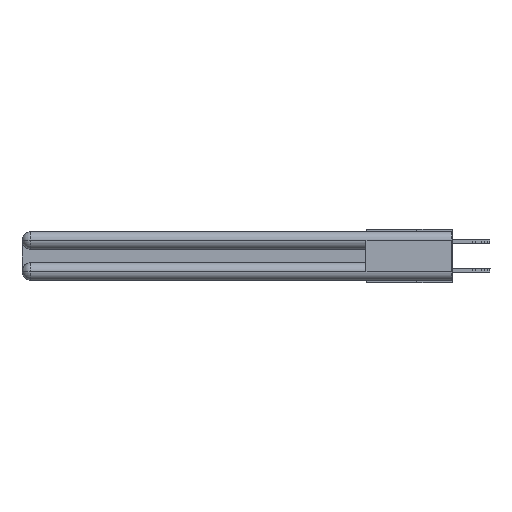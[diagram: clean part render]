
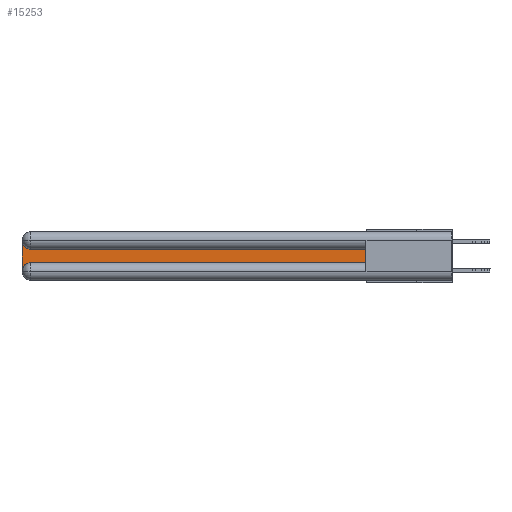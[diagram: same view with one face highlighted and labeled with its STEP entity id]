
A CAD part, left-side view. The second image highlights one B-rep face of the part: STEP entity #15253.
In plain terms, the highlighted planar face has unit normal (-1, 0, 0).
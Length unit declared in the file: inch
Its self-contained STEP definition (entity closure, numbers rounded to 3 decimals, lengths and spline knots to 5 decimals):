
#932 = CARTESIAN_POINT ( 'NONE',  ( 0.075, 2.94, -0.2775 ) ) ;
#955 = PLANE ( 'NONE',  #4731 ) ;
#1133 = EDGE_CURVE ( 'NONE', #23090, #23744, #9291, .T. ) ;
#1704 = LINE ( 'NONE', #3527, #16113 ) ;
#1966 = DIRECTION ( 'NONE',  ( 1., 0., 0. ) ) ;
#3527 = CARTESIAN_POINT ( 'NONE',  ( 0.075, 3., -0.2175 ) ) ;
#3619 = DIRECTION ( 'NONE',  ( 0., 1., 0. ) ) ;
#3834 = CARTESIAN_POINT ( 'NONE',  ( 0.075, 0.6, -0.2175 ) ) ;
#4066 = VERTEX_POINT ( 'NONE', #31238 ) ;
#4229 = VECTOR ( 'NONE', #23165, 39.37008 ) ;
#4731 = AXIS2_PLACEMENT_3D ( 'NONE', #6614, #17396, #9209 ) ;
#5042 = CARTESIAN_POINT ( 'NONE',  ( 0.075, 2.94, -0.1225 ) ) ;
#6614 = CARTESIAN_POINT ( 'NONE',  ( 0.075, 3., -0.1225 ) ) ;
#7005 = VERTEX_POINT ( 'NONE', #5042 ) ;
#7265 = CARTESIAN_POINT ( 'NONE',  ( 0.075, 2.94, -0.0625 ) ) ;
#7665 = AXIS2_PLACEMENT_3D ( 'NONE', #932, #22850, #22621 ) ;
#8088 = VECTOR ( 'NONE', #17691, 39.37008 ) ;
#8724 = EDGE_CURVE ( 'NONE', #25640, #23090, #16023, .T. ) ;
#9209 = DIRECTION ( 'NONE',  ( 0., 0., -1. ) ) ;
#9291 = LINE ( 'NONE', #9478, #4229 ) ;
#9478 = CARTESIAN_POINT ( 'NONE',  ( 0.075, 0.6, -0.2175 ) ) ;
#14307 = VERTEX_POINT ( 'NONE', #34227 ) ;
#14791 = ORIENTED_EDGE ( 'NONE', *, *, #8724, .T. ) ;
#15253 = ADVANCED_FACE ( 'NONE', ( #20458 ), #955, .F. ) ;
#16023 = CIRCLE ( 'NONE', #7665, 0.06 ) ;
#16113 = VECTOR ( 'NONE', #22501, 39.37008 ) ;
#17396 = DIRECTION ( 'NONE',  ( 1., 0., 0. ) ) ;
#17691 = DIRECTION ( 'NONE',  ( 0., 0., 1. ) ) ;
#18171 = ORIENTED_EDGE ( 'NONE', *, *, #1133, .T. ) ;
#19861 = ORIENTED_EDGE ( 'NONE', *, *, #34263, .T. ) ;
#20234 = CARTESIAN_POINT ( 'NONE',  ( 0.075, 0.6, -0.1225 ) ) ;
#20382 = EDGE_LOOP ( 'NONE', ( #28354, #23493, #34566, #14791, #18171, #19861 ) ) ;
#20458 = FACE_OUTER_BOUND ( 'NONE', #20382, .T. ) ;
#20697 = CARTESIAN_POINT ( 'NONE',  ( 0.075, 2.94, -0.2175 ) ) ;
#21465 = CARTESIAN_POINT ( 'NONE',  ( 0.075, 0.6, -0.2175 ) ) ;
#22501 = DIRECTION ( 'NONE',  ( 0., 0., -1. ) ) ;
#22621 = DIRECTION ( 'NONE',  ( 0., 0., -1. ) ) ;
#22850 = DIRECTION ( 'NONE',  ( 1., 0., 0. ) ) ;
#23090 = VERTEX_POINT ( 'NONE', #20697 ) ;
#23165 = DIRECTION ( 'NONE',  ( 0., -1., 0. ) ) ;
#23493 = ORIENTED_EDGE ( 'NONE', *, *, #26730, .T. ) ;
#23744 = VERTEX_POINT ( 'NONE', #21465 ) ;
#24038 = LINE ( 'NONE', #20234, #27482 ) ;
#25271 = CIRCLE ( 'NONE', #31290, 0.06 ) ;
#25640 = VERTEX_POINT ( 'NONE', #32980 ) ;
#26730 = EDGE_CURVE ( 'NONE', #7005, #14307, #25271, .T. ) ;
#27482 = VECTOR ( 'NONE', #3619, 39.37008 ) ;
#28354 = ORIENTED_EDGE ( 'NONE', *, *, #31181, .T. ) ;
#29781 = LINE ( 'NONE', #3834, #8088 ) ;
#31181 = EDGE_CURVE ( 'NONE', #4066, #7005, #24038, .T. ) ;
#31238 = CARTESIAN_POINT ( 'NONE',  ( 0.075, 0.6, -0.1225 ) ) ;
#31290 = AXIS2_PLACEMENT_3D ( 'NONE', #7265, #1966, #31861 ) ;
#31861 = DIRECTION ( 'NONE',  ( 0., 0., -1. ) ) ;
#32980 = CARTESIAN_POINT ( 'NONE',  ( 0.075, 3., -0.2775 ) ) ;
#34227 = CARTESIAN_POINT ( 'NONE',  ( 0.075, 3., -0.0625 ) ) ;
#34263 = EDGE_CURVE ( 'NONE', #23744, #4066, #29781, .T. ) ;
#34566 = ORIENTED_EDGE ( 'NONE', *, *, #34702, .T. ) ;
#34702 = EDGE_CURVE ( 'NONE', #14307, #25640, #1704, .T. ) ;
